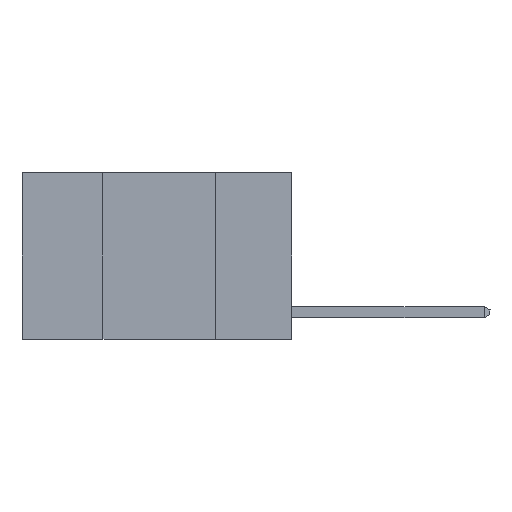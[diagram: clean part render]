
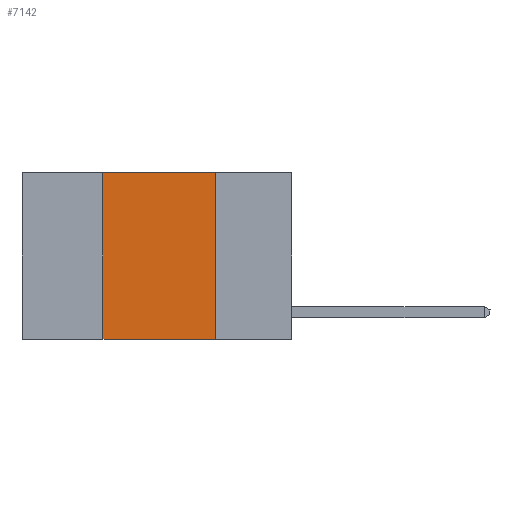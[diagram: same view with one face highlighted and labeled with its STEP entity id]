
A CAD part, left-side view. The second image highlights one B-rep face of the part: STEP entity #7142.
In plain terms, the highlighted planar face has unit normal (-1, 0, 0).
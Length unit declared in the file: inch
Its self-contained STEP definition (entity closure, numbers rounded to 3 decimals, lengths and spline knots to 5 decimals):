
#194 = LINE ( 'NONE', #287, #4978 ) ;
#287 = CARTESIAN_POINT ( 'NONE',  ( 0., 0.42, 0. ) ) ;
#326 = AXIS2_PLACEMENT_3D ( 'NONE', #8657, #7747, #2087 ) ;
#350 = EDGE_CURVE ( 'NONE', #6166, #9606, #194, .T. ) ;
#766 = LINE ( 'NONE', #4607, #11518 ) ;
#792 = VECTOR ( 'NONE', #3066, 39.37008 ) ;
#1157 = PLANE ( 'NONE',  #326 ) ;
#1213 = LINE ( 'NONE', #10556, #11084 ) ;
#1270 = CARTESIAN_POINT ( 'NONE',  ( 0., 0.6, -0.37 ) ) ;
#1450 = EDGE_CURVE ( 'NONE', #6166, #9756, #5272, .T. ) ;
#2087 = DIRECTION ( 'NONE',  ( 0., 0., -1. ) ) ;
#2501 = CARTESIAN_POINT ( 'NONE',  ( 0., 0.42, 0. ) ) ;
#3066 = DIRECTION ( 'NONE',  ( 0., -1., 0. ) ) ;
#3715 = DIRECTION ( 'NONE',  ( 0., 0., -1. ) ) ;
#3767 = CARTESIAN_POINT ( 'NONE',  ( 0., 0.42, -0.37 ) ) ;
#4607 = CARTESIAN_POINT ( 'NONE',  ( 0., 0.17, 0. ) ) ;
#4892 = EDGE_LOOP ( 'NONE', ( #9856, #9749, #6064, #8309 ) ) ;
#4978 = VECTOR ( 'NONE', #10115, 39.37008 ) ;
#5272 = LINE ( 'NONE', #1270, #792 ) ;
#6064 = ORIENTED_EDGE ( 'NONE', *, *, #350, .F. ) ;
#6166 = VERTEX_POINT ( 'NONE', #3767 ) ;
#6582 = EDGE_CURVE ( 'NONE', #9606, #11542, #1213, .T. ) ;
#7142 = ADVANCED_FACE ( 'NONE', ( #10582 ), #1157, .F. ) ;
#7708 = DIRECTION ( 'NONE',  ( 0., -1., 0. ) ) ;
#7747 = DIRECTION ( 'NONE',  ( 1., 0., 0. ) ) ;
#8309 = ORIENTED_EDGE ( 'NONE', *, *, #1450, .T. ) ;
#8657 = CARTESIAN_POINT ( 'NONE',  ( 0., 0.6, 0. ) ) ;
#9389 = CARTESIAN_POINT ( 'NONE',  ( 0., 0.17, 0. ) ) ;
#9606 = VERTEX_POINT ( 'NONE', #2501 ) ;
#9644 = EDGE_CURVE ( 'NONE', #11542, #9756, #766, .T. ) ;
#9749 = ORIENTED_EDGE ( 'NONE', *, *, #6582, .F. ) ;
#9756 = VERTEX_POINT ( 'NONE', #11292 ) ;
#9856 = ORIENTED_EDGE ( 'NONE', *, *, #9644, .F. ) ;
#10115 = DIRECTION ( 'NONE',  ( 0., 0., 1. ) ) ;
#10556 = CARTESIAN_POINT ( 'NONE',  ( 0., 0.6, 0. ) ) ;
#10582 = FACE_OUTER_BOUND ( 'NONE', #4892, .T. ) ;
#11084 = VECTOR ( 'NONE', #7708, 39.37008 ) ;
#11292 = CARTESIAN_POINT ( 'NONE',  ( 0., 0.17, -0.37 ) ) ;
#11518 = VECTOR ( 'NONE', #3715, 39.37008 ) ;
#11542 = VERTEX_POINT ( 'NONE', #9389 ) ;
